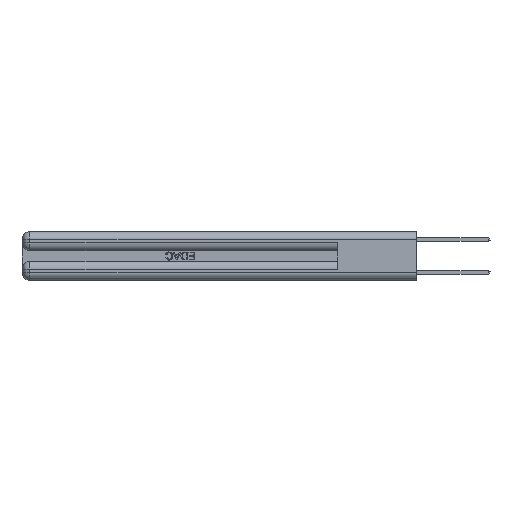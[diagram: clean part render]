
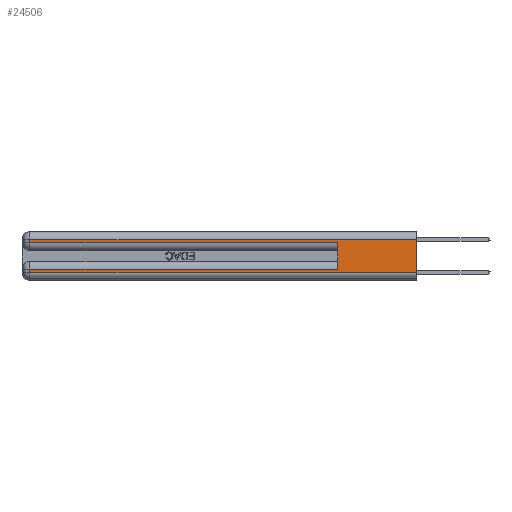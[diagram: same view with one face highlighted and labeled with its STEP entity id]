
A CAD part, left-side view. The second image highlights one B-rep face of the part: STEP entity #24506.
In plain terms, the highlighted planar face has unit normal (-1, 0, 0).
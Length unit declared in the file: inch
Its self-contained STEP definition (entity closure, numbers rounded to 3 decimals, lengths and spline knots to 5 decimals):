
#137 = VERTEX_POINT ( 'NONE', #21883 ) ;
#540 = EDGE_CURVE ( 'NONE', #23062, #1134, #12231, .T. ) ;
#645 = EDGE_CURVE ( 'NONE', #27466, #5244, #2511, .T. ) ;
#1134 = VERTEX_POINT ( 'NONE', #25218 ) ;
#2511 = LINE ( 'NONE', #18304, #28455 ) ;
#3082 = LINE ( 'NONE', #28772, #23826 ) ;
#3650 = ORIENTED_EDGE ( 'NONE', *, *, #32268, .T. ) ;
#4081 = CARTESIAN_POINT ( 'NONE',  ( 0., 0.6, 0.285 ) ) ;
#4641 = CARTESIAN_POINT ( 'NONE',  ( 0., 0., 0.37 ) ) ;
#4832 = PLANE ( 'NONE',  #12300 ) ;
#5244 = VERTEX_POINT ( 'NONE', #4081 ) ;
#7298 = ORIENTED_EDGE ( 'NONE', *, *, #21045, .T. ) ;
#7845 = VECTOR ( 'NONE', #25062, 39.37008 ) ;
#8015 = EDGE_CURVE ( 'NONE', #27001, #23062, #22636, .T. ) ;
#8497 = VERTEX_POINT ( 'NONE', #17494 ) ;
#9079 = EDGE_CURVE ( 'NONE', #13853, #5244, #23995, .T. ) ;
#9176 = DIRECTION ( 'NONE',  ( 0., 1., 0. ) ) ;
#9589 = DIRECTION ( 'NONE',  ( 0., 1., 0. ) ) ;
#9903 = CARTESIAN_POINT ( 'NONE',  ( 0., 0., 0.37 ) ) ;
#12231 = LINE ( 'NONE', #32492, #31101 ) ;
#12300 = AXIS2_PLACEMENT_3D ( 'NONE', #9903, #29695, #14370 ) ;
#13853 = VERTEX_POINT ( 'NONE', #18431 ) ;
#14370 = DIRECTION ( 'NONE',  ( 0., 0., -1. ) ) ;
#14605 = ORIENTED_EDGE ( 'NONE', *, *, #9079, .F. ) ;
#14650 = VECTOR ( 'NONE', #9176, 39.37008 ) ;
#15264 = VECTOR ( 'NONE', #9589, 39.37008 ) ;
#15338 = ORIENTED_EDGE ( 'NONE', *, *, #540, .T. ) ;
#15743 = ORIENTED_EDGE ( 'NONE', *, *, #28696, .T. ) ;
#15938 = DIRECTION ( 'NONE',  ( 0., 0., -1. ) ) ;
#17157 = CARTESIAN_POINT ( 'NONE',  ( 0., 0., 0.085 ) ) ;
#17494 = CARTESIAN_POINT ( 'NONE',  ( 0., 0., 0.31 ) ) ;
#17635 = LINE ( 'NONE', #4641, #7845 ) ;
#18304 = CARTESIAN_POINT ( 'NONE',  ( 0., 0., 0.285 ) ) ;
#18431 = CARTESIAN_POINT ( 'NONE',  ( 0., 0.6, 0.085 ) ) ;
#19790 = FACE_OUTER_BOUND ( 'NONE', #31521, .T. ) ;
#20794 = DIRECTION ( 'NONE',  ( 0., -1., 0. ) ) ;
#21045 = EDGE_CURVE ( 'NONE', #137, #27466, #3082, .T. ) ;
#21508 = CARTESIAN_POINT ( 'NONE',  ( 0., 0.6, 0.145 ) ) ;
#21684 = CARTESIAN_POINT ( 'NONE',  ( 0., 0., 0.31 ) ) ;
#21883 = CARTESIAN_POINT ( 'NONE',  ( 0., 2.94, 0.31 ) ) ;
#22101 = LINE ( 'NONE', #17157, #15264 ) ;
#22611 = VECTOR ( 'NONE', #30381, 39.37008 ) ;
#22636 = LINE ( 'NONE', #25283, #22611 ) ;
#23062 = VERTEX_POINT ( 'NONE', #30214 ) ;
#23826 = VECTOR ( 'NONE', #15938, 39.37008 ) ;
#23995 = LINE ( 'NONE', #21508, #30542 ) ;
#24375 = ORIENTED_EDGE ( 'NONE', *, *, #29098, .F. ) ;
#24506 = ADVANCED_FACE ( 'NONE', ( #19790 ), #4832, .F. ) ;
#25062 = DIRECTION ( 'NONE',  ( 0., 0., -1. ) ) ;
#25218 = CARTESIAN_POINT ( 'NONE',  ( 0., 0., 0.06 ) ) ;
#25283 = CARTESIAN_POINT ( 'NONE',  ( 0., 2.94, 0.37 ) ) ;
#27001 = VERTEX_POINT ( 'NONE', #28073 ) ;
#27466 = VERTEX_POINT ( 'NONE', #27867 ) ;
#27867 = CARTESIAN_POINT ( 'NONE',  ( 0., 2.94, 0.285 ) ) ;
#28073 = CARTESIAN_POINT ( 'NONE',  ( 0., 2.94, 0.085 ) ) ;
#28455 = VECTOR ( 'NONE', #20794, 39.37008 ) ;
#28696 = EDGE_CURVE ( 'NONE', #8497, #137, #32214, .T. ) ;
#28772 = CARTESIAN_POINT ( 'NONE',  ( 0., 2.94, 0.37 ) ) ;
#29098 = EDGE_CURVE ( 'NONE', #8497, #1134, #17635, .T. ) ;
#29695 = DIRECTION ( 'NONE',  ( 1., 0., 0. ) ) ;
#30214 = CARTESIAN_POINT ( 'NONE',  ( 0., 2.94, 0.06 ) ) ;
#30381 = DIRECTION ( 'NONE',  ( 0., 0., -1. ) ) ;
#30542 = VECTOR ( 'NONE', #31561, 39.37008 ) ;
#30599 = ORIENTED_EDGE ( 'NONE', *, *, #8015, .T. ) ;
#31101 = VECTOR ( 'NONE', #32335, 39.37008 ) ;
#31521 = EDGE_LOOP ( 'NONE', ( #24375, #15743, #7298, #32333, #14605, #3650, #30599, #15338 ) ) ;
#31561 = DIRECTION ( 'NONE',  ( 0., 0., 1. ) ) ;
#32214 = LINE ( 'NONE', #21684, #14650 ) ;
#32268 = EDGE_CURVE ( 'NONE', #13853, #27001, #22101, .T. ) ;
#32333 = ORIENTED_EDGE ( 'NONE', *, *, #645, .T. ) ;
#32335 = DIRECTION ( 'NONE',  ( 0., -1., 0. ) ) ;
#32492 = CARTESIAN_POINT ( 'NONE',  ( 0., 0., 0.06 ) ) ;
